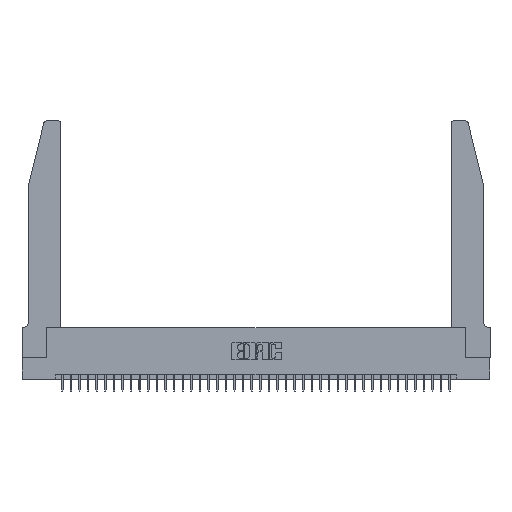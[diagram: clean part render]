
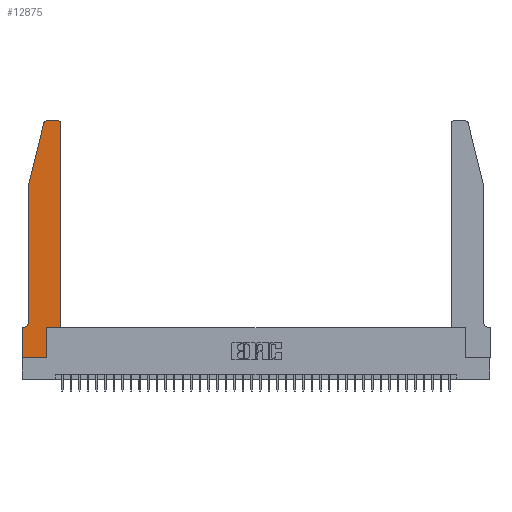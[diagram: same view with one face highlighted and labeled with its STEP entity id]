
A CAD part, top view. The second image highlights one B-rep face of the part: STEP entity #12875.
In plain terms, the highlighted planar face has unit normal (0, 0, 1).
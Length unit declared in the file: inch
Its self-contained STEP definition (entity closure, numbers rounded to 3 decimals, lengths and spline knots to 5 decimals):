
#170 = LINE ( 'NONE', #28001, #11091 ) ;
#430 = EDGE_CURVE ( 'NONE', #21385, #34744, #30899, .T. ) ;
#523 = VECTOR ( 'NONE', #29278, 39.37008 ) ;
#525 = CARTESIAN_POINT ( 'NONE',  ( 0.0055, 0.42, 0.37 ) ) ;
#811 = DIRECTION ( 'NONE',  ( 0., -1., 0. ) ) ;
#930 = CARTESIAN_POINT ( 'NONE',  ( 0.25487, 2.72718, 0.37 ) ) ;
#1064 = CARTESIAN_POINT ( 'NONE',  ( 0.0055, 0.35, 0.37 ) ) ;
#1372 = DIRECTION ( 'NONE',  ( 0., 0., 1. ) ) ;
#1534 = CARTESIAN_POINT ( 'NONE',  ( 0.0755, 2., 0.37 ) ) ;
#1780 = EDGE_CURVE ( 'NONE', #3857, #35332, #31554, .T. ) ;
#2041 = DIRECTION ( 'NONE',  ( -0.239, -0.971, 0. ) ) ;
#2407 = ORIENTED_EDGE ( 'NONE', *, *, #22652, .T. ) ;
#2878 = CARTESIAN_POINT ( 'NONE',  ( 0.4505, 0.35, 0.37 ) ) ;
#2897 = CARTESIAN_POINT ( 'NONE',  ( 0.2865, 0.35, 0.37 ) ) ;
#2997 = DIRECTION ( 'NONE',  ( -1., 0., 0. ) ) ;
#3281 = ORIENTED_EDGE ( 'NONE', *, *, #27180, .T. ) ;
#3523 = EDGE_CURVE ( 'NONE', #24015, #33871, #16069, .T. ) ;
#3527 = DIRECTION ( 'NONE',  ( 1., 0., 0. ) ) ;
#3857 = VERTEX_POINT ( 'NONE', #31463 ) ;
#4703 = CIRCLE ( 'NONE', #12496, 0.07 ) ;
#4940 = VECTOR ( 'NONE', #27829, 39.37008 ) ;
#5111 = EDGE_LOOP ( 'NONE', ( #8309, #29682, #14074, #2407, #3281, #20713, #31106, #16367, #21853, #21777, #31691, #22788 ) ) ;
#5977 = DIRECTION ( 'NONE',  ( 0., 1., 0. ) ) ;
#7587 = CARTESIAN_POINT ( 'NONE',  ( 0.0755, 0.35, 0.37 ) ) ;
#7686 = VECTOR ( 'NONE', #2041, 39.37008 ) ;
#7705 = EDGE_CURVE ( 'NONE', #19965, #38744, #29314, .T. ) ;
#8309 = ORIENTED_EDGE ( 'NONE', *, *, #27422, .T. ) ;
#8624 = VECTOR ( 'NONE', #11937, 39.37008 ) ;
#10113 = VECTOR ( 'NONE', #3527, 39.37008 ) ;
#10377 = PLANE ( 'NONE',  #13222 ) ;
#10723 = EDGE_CURVE ( 'NONE', #11342, #3857, #22488, .T. ) ;
#10941 = DIRECTION ( 'NONE',  ( 0., -1., 0. ) ) ;
#11091 = VECTOR ( 'NONE', #29162, 39.37008 ) ;
#11342 = VERTEX_POINT ( 'NONE', #17111 ) ;
#11636 = CARTESIAN_POINT ( 'NONE',  ( 0.0755, 2., 0.37 ) ) ;
#11750 = VECTOR ( 'NONE', #5977, 39.37008 ) ;
#11937 = DIRECTION ( 'NONE',  ( -1., 0., 0. ) ) ;
#12496 = AXIS2_PLACEMENT_3D ( 'NONE', #525, #37957, #2997 ) ;
#12875 = ADVANCED_FACE ( 'NONE', ( #38415 ), #10377, .T. ) ;
#13222 = AXIS2_PLACEMENT_3D ( 'NONE', #32275, #1372, #22859 ) ;
#13486 = DIRECTION ( 'NONE',  ( 0., 0., 1. ) ) ;
#14074 = ORIENTED_EDGE ( 'NONE', *, *, #37000, .T. ) ;
#14925 = AXIS2_PLACEMENT_3D ( 'NONE', #38558, #35690, #19318 ) ;
#16069 = CIRCLE ( 'NONE', #38953, 0.03 ) ;
#16367 = ORIENTED_EDGE ( 'NONE', *, *, #1780, .T. ) ;
#16401 = CARTESIAN_POINT ( 'NONE',  ( 0., 0., 0.37 ) ) ;
#16956 = CARTESIAN_POINT ( 'NONE',  ( 0.4205, 2.72, 0.37 ) ) ;
#17111 = CARTESIAN_POINT ( 'NONE',  ( 0., 0.35, 0.37 ) ) ;
#18139 = CARTESIAN_POINT ( 'NONE',  ( 0.4505, 2.72, 0.37 ) ) ;
#18432 = LINE ( 'NONE', #2897, #11750 ) ;
#19318 = DIRECTION ( 'NONE',  ( 1., 0., 0. ) ) ;
#19965 = VERTEX_POINT ( 'NONE', #36025 ) ;
#20558 = CARTESIAN_POINT ( 'NONE',  ( 0.2605, 2.75, 0.37 ) ) ;
#20713 = ORIENTED_EDGE ( 'NONE', *, *, #39534, .T. ) ;
#21385 = VERTEX_POINT ( 'NONE', #38843 ) ;
#21777 = ORIENTED_EDGE ( 'NONE', *, *, #430, .T. ) ;
#21853 = ORIENTED_EDGE ( 'NONE', *, *, #23060, .T. ) ;
#22394 = EDGE_CURVE ( 'NONE', #34744, #24015, #170, .T. ) ;
#22488 = LINE ( 'NONE', #31916, #34679 ) ;
#22652 = EDGE_CURVE ( 'NONE', #36035, #29866, #29568, .T. ) ;
#22788 = ORIENTED_EDGE ( 'NONE', *, *, #3523, .T. ) ;
#22857 = VECTOR ( 'NONE', #10941, 39.37008 ) ;
#22859 = DIRECTION ( 'NONE',  ( 1., 0., 0. ) ) ;
#23060 = EDGE_CURVE ( 'NONE', #35332, #21385, #18432, .T. ) ;
#23621 = LINE ( 'NONE', #20558, #8624 ) ;
#23856 = CARTESIAN_POINT ( 'NONE',  ( 0.0755, 2., 0.37 ) ) ;
#24015 = VERTEX_POINT ( 'NONE', #18139 ) ;
#25982 = DIRECTION ( 'NONE',  ( 1., 0., 0. ) ) ;
#27180 = EDGE_CURVE ( 'NONE', #29866, #33594, #4703, .T. ) ;
#27422 = EDGE_CURVE ( 'NONE', #33871, #19965, #23621, .T. ) ;
#27829 = DIRECTION ( 'NONE',  ( 1., 0., 0. ) ) ;
#28001 = CARTESIAN_POINT ( 'NONE',  ( 0.4505, 0.35, 0.37 ) ) ;
#29162 = DIRECTION ( 'NONE',  ( 0., 1., 0. ) ) ;
#29278 = DIRECTION ( 'NONE',  ( -1., 0., 0. ) ) ;
#29314 = CIRCLE ( 'NONE', #14925, 0.03 ) ;
#29568 = LINE ( 'NONE', #1534, #22857 ) ;
#29682 = ORIENTED_EDGE ( 'NONE', *, *, #7705, .T. ) ;
#29866 = VERTEX_POINT ( 'NONE', #37586 ) ;
#30062 = LINE ( 'NONE', #11636, #7686 ) ;
#30899 = LINE ( 'NONE', #2878, #4940 ) ;
#31106 = ORIENTED_EDGE ( 'NONE', *, *, #10723, .T. ) ;
#31463 = CARTESIAN_POINT ( 'NONE',  ( 0., 0., 0.37 ) ) ;
#31554 = LINE ( 'NONE', #16401, #10113 ) ;
#31691 = ORIENTED_EDGE ( 'NONE', *, *, #22394, .T. ) ;
#31916 = CARTESIAN_POINT ( 'NONE',  ( 0., 0., 0.37 ) ) ;
#32275 = CARTESIAN_POINT ( 'NONE',  ( 0., 0.35, 0.37 ) ) ;
#32345 = LINE ( 'NONE', #7587, #523 ) ;
#33594 = VERTEX_POINT ( 'NONE', #1064 ) ;
#33871 = VERTEX_POINT ( 'NONE', #35630 ) ;
#34679 = VECTOR ( 'NONE', #811, 39.37008 ) ;
#34744 = VERTEX_POINT ( 'NONE', #36097 ) ;
#35332 = VERTEX_POINT ( 'NONE', #40111 ) ;
#35630 = CARTESIAN_POINT ( 'NONE',  ( 0.4205, 2.75, 0.37 ) ) ;
#35690 = DIRECTION ( 'NONE',  ( 0., 0., 1. ) ) ;
#36025 = CARTESIAN_POINT ( 'NONE',  ( 0.284, 2.75, 0.37 ) ) ;
#36035 = VERTEX_POINT ( 'NONE', #23856 ) ;
#36097 = CARTESIAN_POINT ( 'NONE',  ( 0.4505, 0.35, 0.37 ) ) ;
#37000 = EDGE_CURVE ( 'NONE', #38744, #36035, #30062, .T. ) ;
#37586 = CARTESIAN_POINT ( 'NONE',  ( 0.0755, 0.42, 0.37 ) ) ;
#37957 = DIRECTION ( 'NONE',  ( 0., 0., -1. ) ) ;
#38415 = FACE_OUTER_BOUND ( 'NONE', #5111, .T. ) ;
#38558 = CARTESIAN_POINT ( 'NONE',  ( 0.284, 2.72, 0.37 ) ) ;
#38744 = VERTEX_POINT ( 'NONE', #930 ) ;
#38843 = CARTESIAN_POINT ( 'NONE',  ( 0.2865, 0.35, 0.37 ) ) ;
#38953 = AXIS2_PLACEMENT_3D ( 'NONE', #16956, #13486, #25982 ) ;
#39534 = EDGE_CURVE ( 'NONE', #33594, #11342, #32345, .T. ) ;
#40111 = CARTESIAN_POINT ( 'NONE',  ( 0.2865, 0., 0.37 ) ) ;
